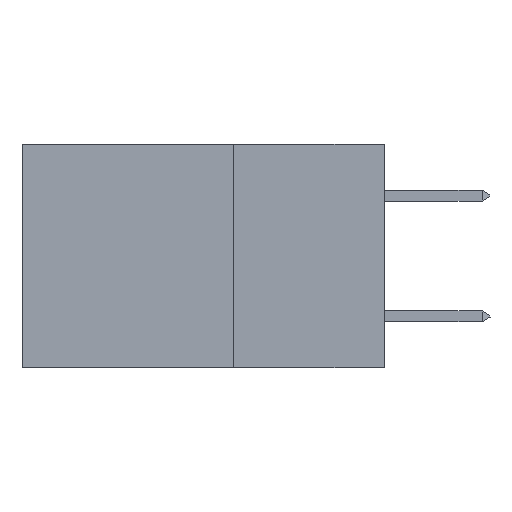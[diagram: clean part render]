
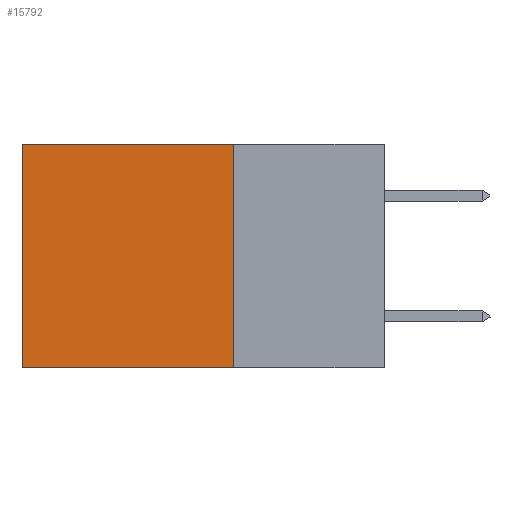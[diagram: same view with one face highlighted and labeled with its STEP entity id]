
A CAD part, left-side view. The second image highlights one B-rep face of the part: STEP entity #15792.
In plain terms, the highlighted planar face has unit normal (-1, 0, 0).
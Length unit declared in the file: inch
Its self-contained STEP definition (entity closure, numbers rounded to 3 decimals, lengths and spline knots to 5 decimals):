
#10 = VECTOR ( 'NONE', #1204, 39.37008 ) ;
#79 = DIRECTION ( 'NONE',  ( 0., 1., 0. ) ) ;
#457 = DIRECTION ( 'NONE',  ( 0., 0., -1. ) ) ;
#1165 = ORIENTED_EDGE ( 'NONE', *, *, #11308, .T. ) ;
#1204 = DIRECTION ( 'NONE',  ( 0., 1., 0. ) ) ;
#2229 = VECTOR ( 'NONE', #8518, 39.37008 ) ;
#2319 = CARTESIAN_POINT ( 'NONE',  ( 0.2875, 0.6, -0.37 ) ) ;
#2445 = AXIS2_PLACEMENT_3D ( 'NONE', #9136, #16336, #10778 ) ;
#2512 = LINE ( 'NONE', #7503, #16043 ) ;
#2717 = VERTEX_POINT ( 'NONE', #2319 ) ;
#2766 = LINE ( 'NONE', #7373, #6138 ) ;
#3396 = CARTESIAN_POINT ( 'NONE',  ( 0.2875, 0.6, 0. ) ) ;
#5424 = ORIENTED_EDGE ( 'NONE', *, *, #14819, .T. ) ;
#6138 = VECTOR ( 'NONE', #79, 39.37008 ) ;
#6403 = EDGE_CURVE ( 'NONE', #11154, #2717, #9018, .T. ) ;
#7373 = CARTESIAN_POINT ( 'NONE',  ( 0.2875, 0.25, 0. ) ) ;
#7503 = CARTESIAN_POINT ( 'NONE',  ( 0.2875, 0.25, 0. ) ) ;
#8518 = DIRECTION ( 'NONE',  ( 0., 0., -1. ) ) ;
#9018 = LINE ( 'NONE', #10319, #10 ) ;
#9136 = CARTESIAN_POINT ( 'NONE',  ( 0.2875, 0.25, 0. ) ) ;
#10319 = CARTESIAN_POINT ( 'NONE',  ( 0.2875, 0.25, -0.37 ) ) ;
#10544 = CARTESIAN_POINT ( 'NONE',  ( 0.2875, 0.25, 0. ) ) ;
#10778 = DIRECTION ( 'NONE',  ( 0., 0., -1. ) ) ;
#11154 = VERTEX_POINT ( 'NONE', #12496 ) ;
#11308 = EDGE_CURVE ( 'NONE', #13270, #2717, #17343, .T. ) ;
#12496 = CARTESIAN_POINT ( 'NONE',  ( 0.2875, 0.25, -0.37 ) ) ;
#12738 = CARTESIAN_POINT ( 'NONE',  ( 0.2875, 0.6, 0. ) ) ;
#13270 = VERTEX_POINT ( 'NONE', #3396 ) ;
#13789 = VERTEX_POINT ( 'NONE', #10544 ) ;
#14245 = ORIENTED_EDGE ( 'NONE', *, *, #15635, .F. ) ;
#14644 = ORIENTED_EDGE ( 'NONE', *, *, #6403, .F. ) ;
#14819 = EDGE_CURVE ( 'NONE', #13789, #13270, #2766, .T. ) ;
#15635 = EDGE_CURVE ( 'NONE', #13789, #11154, #2512, .T. ) ;
#15792 = ADVANCED_FACE ( 'NONE', ( #17392 ), #16460, .F. ) ;
#16043 = VECTOR ( 'NONE', #457, 39.37008 ) ;
#16132 = EDGE_LOOP ( 'NONE', ( #1165, #14644, #14245, #5424 ) ) ;
#16336 = DIRECTION ( 'NONE',  ( 1., 0., 0. ) ) ;
#16460 = PLANE ( 'NONE',  #2445 ) ;
#17343 = LINE ( 'NONE', #12738, #2229 ) ;
#17392 = FACE_OUTER_BOUND ( 'NONE', #16132, .T. ) ;
